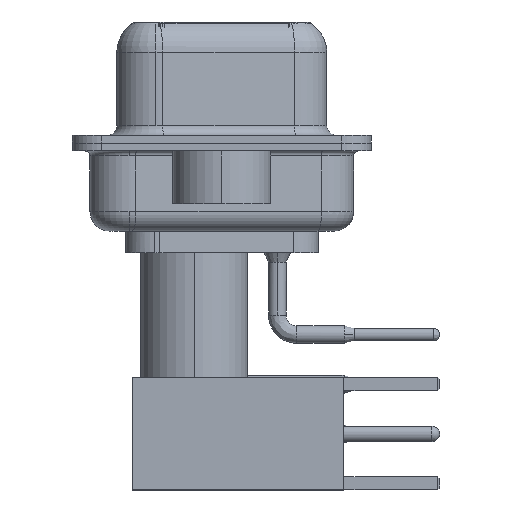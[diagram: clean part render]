
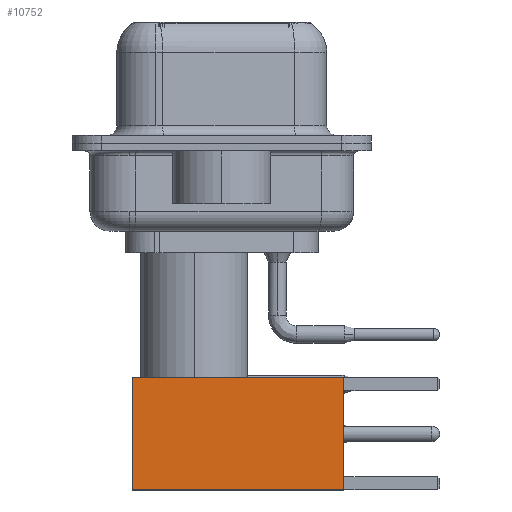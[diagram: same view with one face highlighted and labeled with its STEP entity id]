
A CAD part, left-side view. The second image highlights one B-rep face of the part: STEP entity #10752.
In plain terms, the highlighted face is planar.
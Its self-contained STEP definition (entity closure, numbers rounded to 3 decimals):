
#1325 = CARTESIAN_POINT ( 'NONE',  ( 0., 2.875, 0. ) ) ;
#2577 = VERTEX_POINT ( 'NONE', #37033 ) ;
#3453 = EDGE_CURVE ( 'NONE', #28488, #4753, #7124, .T. ) ;
#4753 = VERTEX_POINT ( 'NONE', #9633 ) ;
#4768 = AXIS2_PLACEMENT_3D ( 'NONE', #21674, #22049, #33278 ) ;
#5487 = CARTESIAN_POINT ( 'NONE',  ( -2.875, 2.875, 0. ) ) ;
#7124 = LINE ( 'NONE', #1325, #16799 ) ;
#7930 = LINE ( 'NONE', #21812, #32238 ) ;
#9633 = CARTESIAN_POINT ( 'NONE',  ( -2.875, 2.875, 0. ) ) ;
#9813 = EDGE_CURVE ( 'NONE', #2577, #28488, #7930, .T. ) ;
#10248 = FACE_OUTER_BOUND ( 'NONE', #19335, .T. ) ;
#10752 = ADVANCED_FACE ( 'NONE', ( #10248 ), #30292, .T. ) ;
#11082 = ORIENTED_EDGE ( 'NONE', *, *, #3453, .T. ) ;
#12370 = CARTESIAN_POINT ( 'NONE',  ( 2.875, 2.875, 0. ) ) ;
#13998 = VERTEX_POINT ( 'NONE', #22853 ) ;
#14206 = VECTOR ( 'NONE', #17140, 1000. ) ;
#16741 = LINE ( 'NONE', #5487, #26358 ) ;
#16799 = VECTOR ( 'NONE', #18564, 1000. ) ;
#17140 = DIRECTION ( 'NONE',  ( -1., 0., 0. ) ) ;
#17324 = CARTESIAN_POINT ( 'NONE',  ( 0., 2.875, 10.82 ) ) ;
#18564 = DIRECTION ( 'NONE',  ( -1., 0., 0. ) ) ;
#19335 = EDGE_LOOP ( 'NONE', ( #22839, #11082, #32865, #23918 ) ) ;
#19541 = LINE ( 'NONE', #17324, #14206 ) ;
#21674 = CARTESIAN_POINT ( 'NONE',  ( 2.875, 2.875, 0. ) ) ;
#21812 = CARTESIAN_POINT ( 'NONE',  ( 2.875, 2.875, 0. ) ) ;
#21905 = EDGE_CURVE ( 'NONE', #2577, #13998, #19541, .T. ) ;
#22049 = DIRECTION ( 'NONE',  ( 0., 1., 0. ) ) ;
#22731 = DIRECTION ( 'NONE',  ( 0., 0., -1. ) ) ;
#22839 = ORIENTED_EDGE ( 'NONE', *, *, #9813, .T. ) ;
#22853 = CARTESIAN_POINT ( 'NONE',  ( -2.875, 2.875, 10.82 ) ) ;
#23918 = ORIENTED_EDGE ( 'NONE', *, *, #21905, .F. ) ;
#26358 = VECTOR ( 'NONE', #22731, 1000. ) ;
#28488 = VERTEX_POINT ( 'NONE', #12370 ) ;
#30292 = PLANE ( 'NONE',  #4768 ) ;
#32238 = VECTOR ( 'NONE', #32852, 1000. ) ;
#32852 = DIRECTION ( 'NONE',  ( 0., 0., -1. ) ) ;
#32865 = ORIENTED_EDGE ( 'NONE', *, *, #33445, .F. ) ;
#33278 = DIRECTION ( 'NONE',  ( 0., 0., 1. ) ) ;
#33445 = EDGE_CURVE ( 'NONE', #13998, #4753, #16741, .T. ) ;
#37033 = CARTESIAN_POINT ( 'NONE',  ( 2.875, 2.875, 10.82 ) ) ;
